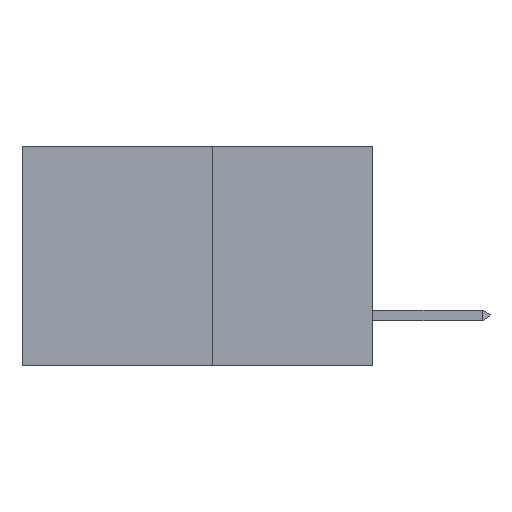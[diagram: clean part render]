
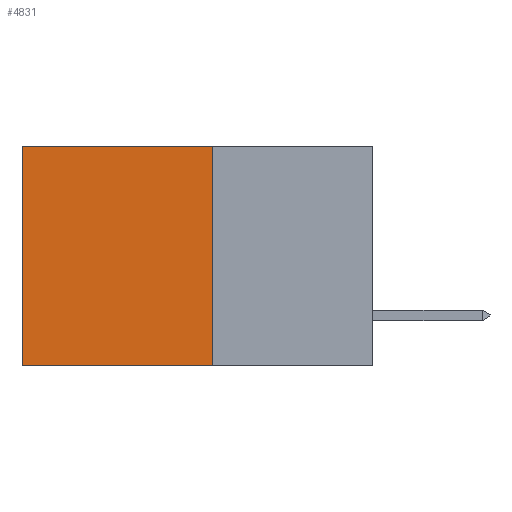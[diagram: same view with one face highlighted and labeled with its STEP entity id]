
A CAD part, left-side view. The second image highlights one B-rep face of the part: STEP entity #4831.
In plain terms, the highlighted planar face has unit normal (-1, 0, 0).
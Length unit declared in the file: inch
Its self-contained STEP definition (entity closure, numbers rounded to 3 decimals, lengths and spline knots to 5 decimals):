
#2115 = CARTESIAN_POINT ( 'NONE',  ( 0.277, 0.27, -0.37 ) ) ;
#2199 = ORIENTED_EDGE ( 'NONE', *, *, #21946, .F. ) ;
#2759 = EDGE_CURVE ( 'NONE', #12218, #17802, #16437, .T. ) ;
#2970 = AXIS2_PLACEMENT_3D ( 'NONE', #2115, #14771, #3980 ) ;
#3461 = ORIENTED_EDGE ( 'NONE', *, *, #2759, .T. ) ;
#3901 = PLANE ( 'NONE',  #2970 ) ;
#3980 = DIRECTION ( 'NONE',  ( 0., 0., -1. ) ) ;
#4442 = DIRECTION ( 'NONE',  ( 0., 1., 0. ) ) ;
#4831 = ADVANCED_FACE ( 'NONE', ( #13027 ), #3901, .F. ) ;
#5530 = EDGE_CURVE ( 'NONE', #18454, #12218, #14394, .T. ) ;
#6920 = VECTOR ( 'NONE', #18458, 39.37008 ) ;
#8023 = CARTESIAN_POINT ( 'NONE',  ( 0.277, 0.59, 0. ) ) ;
#8027 = CARTESIAN_POINT ( 'NONE',  ( 0.277, 0.27, 0. ) ) ;
#8264 = VECTOR ( 'NONE', #4442, 39.37008 ) ;
#8537 = ORIENTED_EDGE ( 'NONE', *, *, #16203, .F. ) ;
#10024 = CARTESIAN_POINT ( 'NONE',  ( 0.277, 0.27, -0.37 ) ) ;
#11104 = DIRECTION ( 'NONE',  ( 0., 0., -1. ) ) ;
#12218 = VERTEX_POINT ( 'NONE', #8023 ) ;
#12318 = ORIENTED_EDGE ( 'NONE', *, *, #5530, .T. ) ;
#12907 = CARTESIAN_POINT ( 'NONE',  ( 0.277, 0.27, -0.37 ) ) ;
#13027 = FACE_OUTER_BOUND ( 'NONE', #16133, .T. ) ;
#13266 = VECTOR ( 'NONE', #18352, 39.37008 ) ;
#14394 = LINE ( 'NONE', #16450, #13266 ) ;
#14771 = DIRECTION ( 'NONE',  ( 1., 0., 0. ) ) ;
#14785 = LINE ( 'NONE', #12907, #18437 ) ;
#15129 = CARTESIAN_POINT ( 'NONE',  ( 0.277, 0.27, -0.37 ) ) ;
#16133 = EDGE_LOOP ( 'NONE', ( #3461, #2199, #8537, #12318 ) ) ;
#16203 = EDGE_CURVE ( 'NONE', #18454, #17692, #14785, .T. ) ;
#16437 = LINE ( 'NONE', #18160, #6920 ) ;
#16450 = CARTESIAN_POINT ( 'NONE',  ( 0.277, 0.27, 0. ) ) ;
#17515 = CARTESIAN_POINT ( 'NONE',  ( 0.277, 0.59, -0.37 ) ) ;
#17692 = VERTEX_POINT ( 'NONE', #10024 ) ;
#17802 = VERTEX_POINT ( 'NONE', #17515 ) ;
#18160 = CARTESIAN_POINT ( 'NONE',  ( 0.277, 0.59, -0.37 ) ) ;
#18352 = DIRECTION ( 'NONE',  ( 0., 1., 0. ) ) ;
#18437 = VECTOR ( 'NONE', #11104, 39.37008 ) ;
#18454 = VERTEX_POINT ( 'NONE', #8027 ) ;
#18458 = DIRECTION ( 'NONE',  ( 0., 0., -1. ) ) ;
#21471 = LINE ( 'NONE', #15129, #8264 ) ;
#21946 = EDGE_CURVE ( 'NONE', #17692, #17802, #21471, .T. ) ;
